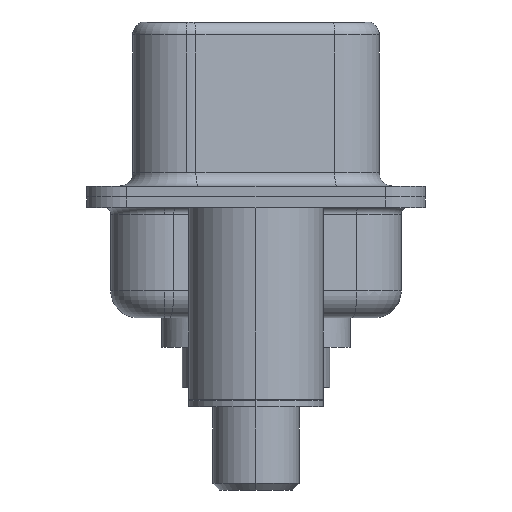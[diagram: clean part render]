
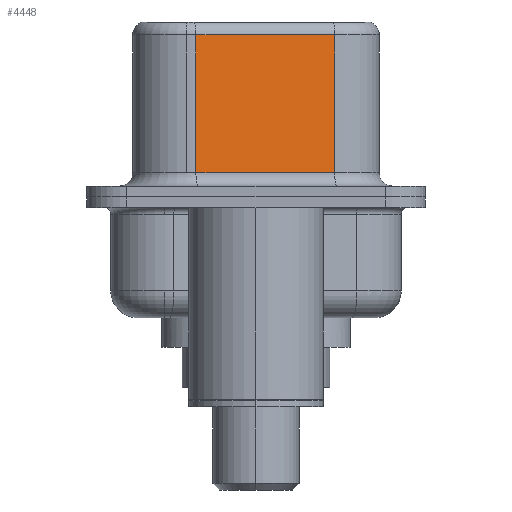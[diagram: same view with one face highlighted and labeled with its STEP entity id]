
A CAD part, left-side view. The second image highlights one B-rep face of the part: STEP entity #4448.
In plain terms, the highlighted planar face has unit normal (-0.985, -0.174, 0).
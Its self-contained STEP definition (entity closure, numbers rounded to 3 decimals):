
#464 = EDGE_LOOP ( 'NONE', ( #4161, #17535, #10352, #10321 ) ) ;
#1062 = CARTESIAN_POINT ( 'NONE',  ( 4.58, -2.927, 6.02 ) ) ;
#1270 = CARTESIAN_POINT ( 'NONE',  ( 3.67, 2.233, 0.9 ) ) ;
#1633 = DIRECTION ( 'NONE',  ( 0.174, -0.985, 0. ) ) ;
#1704 = CARTESIAN_POINT ( 'NONE',  ( 4.58, -2.927, 0.9 ) ) ;
#2444 = VERTEX_POINT ( 'NONE', #1270 ) ;
#2538 = DIRECTION ( 'NONE',  ( 0., 0., -1. ) ) ;
#2619 = CARTESIAN_POINT ( 'NONE',  ( 4.58, -2.927, 6.52 ) ) ;
#3197 = LINE ( 'NONE', #2619, #10370 ) ;
#3888 = VERTEX_POINT ( 'NONE', #8782 ) ;
#4139 = VECTOR ( 'NONE', #6695, 1000. ) ;
#4161 = ORIENTED_EDGE ( 'NONE', *, *, #5626, .F. ) ;
#4448 = ADVANCED_FACE ( 'NONE', ( #10854 ), #6760, .F. ) ;
#4938 = CARTESIAN_POINT ( 'NONE',  ( 4.58, -2.927, 6.52 ) ) ;
#5503 = EDGE_CURVE ( 'NONE', #9858, #2444, #8364, .T. ) ;
#5626 = EDGE_CURVE ( 'NONE', #3888, #10026, #3197, .T. ) ;
#5630 = EDGE_CURVE ( 'NONE', #2444, #10026, #6590, .T. ) ;
#6206 = DIRECTION ( 'NONE',  ( -0.174, 0.985, 0. ) ) ;
#6278 = CARTESIAN_POINT ( 'NONE',  ( 4.58, -2.927, 0.9 ) ) ;
#6516 = DIRECTION ( 'NONE',  ( 0.985, 0.174, 0. ) ) ;
#6535 = CARTESIAN_POINT ( 'NONE',  ( 3.67, 2.233, 6.52 ) ) ;
#6590 = LINE ( 'NONE', #1704, #13764 ) ;
#6695 = DIRECTION ( 'NONE',  ( 0., 0., -1. ) ) ;
#6760 = PLANE ( 'NONE',  #14531 ) ;
#7751 = EDGE_CURVE ( 'NONE', #3888, #9858, #9619, .T. ) ;
#8172 = DIRECTION ( 'NONE',  ( -0.174, 0.985, 0. ) ) ;
#8364 = LINE ( 'NONE', #6535, #4139 ) ;
#8782 = CARTESIAN_POINT ( 'NONE',  ( 4.58, -2.927, 6.02 ) ) ;
#9619 = LINE ( 'NONE', #1062, #16288 ) ;
#9858 = VERTEX_POINT ( 'NONE', #13005 ) ;
#10026 = VERTEX_POINT ( 'NONE', #6278 ) ;
#10321 = ORIENTED_EDGE ( 'NONE', *, *, #5630, .T. ) ;
#10352 = ORIENTED_EDGE ( 'NONE', *, *, #5503, .T. ) ;
#10370 = VECTOR ( 'NONE', #2538, 1000. ) ;
#10854 = FACE_OUTER_BOUND ( 'NONE', #464, .T. ) ;
#13005 = CARTESIAN_POINT ( 'NONE',  ( 3.67, 2.233, 6.02 ) ) ;
#13764 = VECTOR ( 'NONE', #1633, 1000. ) ;
#14531 = AXIS2_PLACEMENT_3D ( 'NONE', #4938, #6516, #6206 ) ;
#16288 = VECTOR ( 'NONE', #8172, 1000. ) ;
#17535 = ORIENTED_EDGE ( 'NONE', *, *, #7751, .T. ) ;
